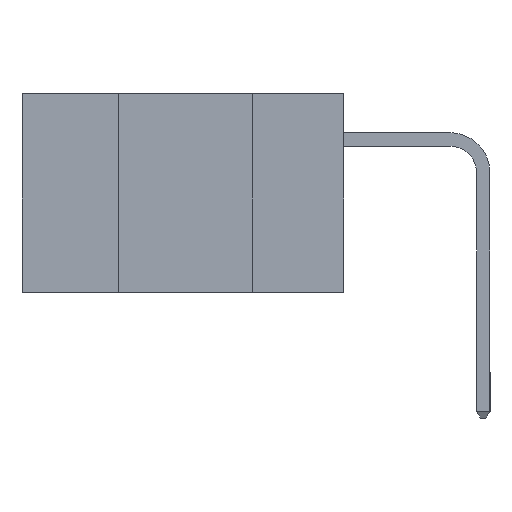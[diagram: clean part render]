
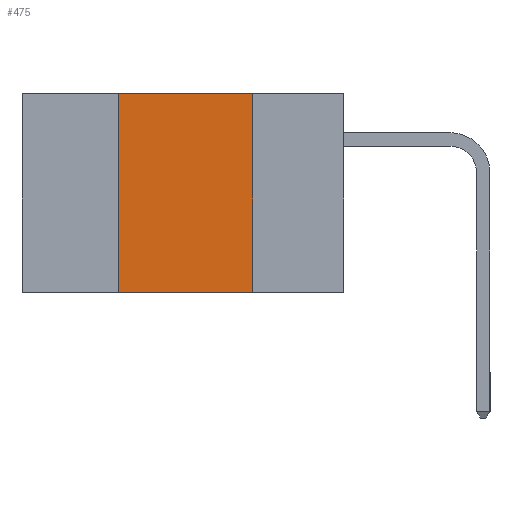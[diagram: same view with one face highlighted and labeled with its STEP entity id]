
A CAD part, left-side view. The second image highlights one B-rep face of the part: STEP entity #475.
In plain terms, the highlighted planar face has unit normal (-1, 0, 0).
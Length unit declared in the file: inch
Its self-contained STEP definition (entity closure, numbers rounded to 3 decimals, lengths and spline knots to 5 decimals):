
#11 = CARTESIAN_POINT ( 'NONE',  ( 0., 0.42, 0. ) ) ;
#475 = ADVANCED_FACE ( 'NONE', ( #17044 ), #1668, .F. ) ;
#756 = EDGE_CURVE ( 'NONE', #2784, #6260, #12278, .T. ) ;
#962 = VECTOR ( 'NONE', #3101, 39.37008 ) ;
#998 = AXIS2_PLACEMENT_3D ( 'NONE', #7175, #9987, #14417 ) ;
#1386 = DIRECTION ( 'NONE',  ( 0., 0., 1. ) ) ;
#1668 = PLANE ( 'NONE',  #998 ) ;
#2784 = VERTEX_POINT ( 'NONE', #16428 ) ;
#3101 = DIRECTION ( 'NONE',  ( 0., 0., -1. ) ) ;
#4109 = ORIENTED_EDGE ( 'NONE', *, *, #17568, .F. ) ;
#5015 = CARTESIAN_POINT ( 'NONE',  ( 0., 0.6, 0. ) ) ;
#5386 = LINE ( 'NONE', #12462, #11012 ) ;
#5914 = ORIENTED_EDGE ( 'NONE', *, *, #9834, .F. ) ;
#6260 = VERTEX_POINT ( 'NONE', #7200 ) ;
#7175 = CARTESIAN_POINT ( 'NONE',  ( 0., 0.6, 0. ) ) ;
#7200 = CARTESIAN_POINT ( 'NONE',  ( 0., 0.17, -0.37 ) ) ;
#7708 = ORIENTED_EDGE ( 'NONE', *, *, #12903, .F. ) ;
#8420 = EDGE_LOOP ( 'NONE', ( #4109, #5914, #7708, #17224 ) ) ;
#8440 = VECTOR ( 'NONE', #13933, 39.37008 ) ;
#8611 = CARTESIAN_POINT ( 'NONE',  ( 0., 0.17, -0.37 ) ) ;
#9080 = VECTOR ( 'NONE', #12271, 39.37008 ) ;
#9834 = EDGE_CURVE ( 'NONE', #10658, #18189, #13489, .T. ) ;
#9987 = DIRECTION ( 'NONE',  ( 1., 0., 0. ) ) ;
#10623 = CARTESIAN_POINT ( 'NONE',  ( 0., 0.17, 0. ) ) ;
#10658 = VERTEX_POINT ( 'NONE', #11 ) ;
#11012 = VECTOR ( 'NONE', #1386, 39.37008 ) ;
#12271 = DIRECTION ( 'NONE',  ( 0., -1., 0. ) ) ;
#12278 = LINE ( 'NONE', #15338, #8440 ) ;
#12462 = CARTESIAN_POINT ( 'NONE',  ( 0., 0.42, -0.37 ) ) ;
#12903 = EDGE_CURVE ( 'NONE', #2784, #10658, #5386, .T. ) ;
#13489 = LINE ( 'NONE', #5015, #9080 ) ;
#13933 = DIRECTION ( 'NONE',  ( 0., -1., 0. ) ) ;
#14417 = DIRECTION ( 'NONE',  ( 0., 0., -1. ) ) ;
#15338 = CARTESIAN_POINT ( 'NONE',  ( 0., 0.6, -0.37 ) ) ;
#16428 = CARTESIAN_POINT ( 'NONE',  ( 0., 0.42, -0.37 ) ) ;
#17044 = FACE_OUTER_BOUND ( 'NONE', #8420, .T. ) ;
#17224 = ORIENTED_EDGE ( 'NONE', *, *, #756, .T. ) ;
#17444 = LINE ( 'NONE', #8611, #962 ) ;
#17568 = EDGE_CURVE ( 'NONE', #18189, #6260, #17444, .T. ) ;
#18189 = VERTEX_POINT ( 'NONE', #10623 ) ;
